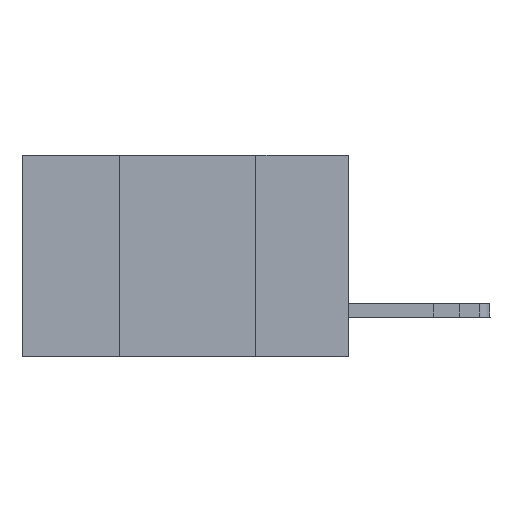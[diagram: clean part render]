
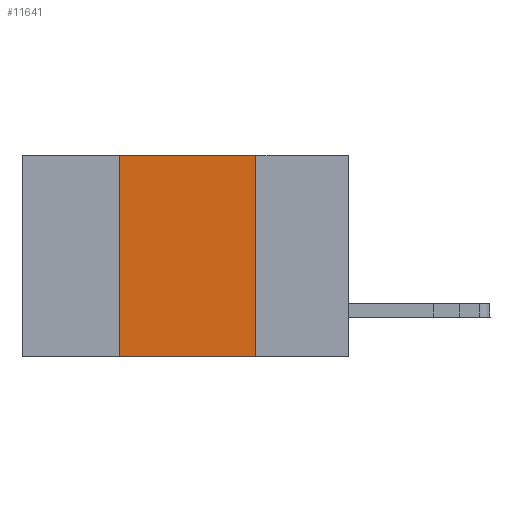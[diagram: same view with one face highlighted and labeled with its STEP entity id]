
A CAD part, left-side view. The second image highlights one B-rep face of the part: STEP entity #11641.
In plain terms, the highlighted planar face has unit normal (-1, 0, 0).
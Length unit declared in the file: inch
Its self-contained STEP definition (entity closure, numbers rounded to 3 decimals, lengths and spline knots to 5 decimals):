
#175 = ORIENTED_EDGE ( 'NONE', *, *, #22905, .F. ) ;
#768 = CARTESIAN_POINT ( 'NONE',  ( 0., 0.6, -0.37 ) ) ;
#1078 = VERTEX_POINT ( 'NONE', #2141 ) ;
#1504 = CARTESIAN_POINT ( 'NONE',  ( 0., 0.42, 0. ) ) ;
#1736 = ORIENTED_EDGE ( 'NONE', *, *, #4784, .T. ) ;
#2096 = PLANE ( 'NONE',  #23273 ) ;
#2141 = CARTESIAN_POINT ( 'NONE',  ( 0., 0.17, 0. ) ) ;
#2751 = VECTOR ( 'NONE', #10337, 39.37008 ) ;
#4326 = CARTESIAN_POINT ( 'NONE',  ( 0., 0.42, -0.37 ) ) ;
#4784 = EDGE_CURVE ( 'NONE', #15627, #7791, #23491, .T. ) ;
#4946 = EDGE_CURVE ( 'NONE', #1078, #7791, #5081, .T. ) ;
#5081 = LINE ( 'NONE', #23608, #14709 ) ;
#5235 = VECTOR ( 'NONE', #21622, 39.37008 ) ;
#6411 = ORIENTED_EDGE ( 'NONE', *, *, #6526, .F. ) ;
#6526 = EDGE_CURVE ( 'NONE', #13753, #1078, #7897, .T. ) ;
#7791 = VERTEX_POINT ( 'NONE', #24075 ) ;
#7897 = LINE ( 'NONE', #15511, #5235 ) ;
#8139 = CARTESIAN_POINT ( 'NONE',  ( 0., 0.6, 0. ) ) ;
#9649 = DIRECTION ( 'NONE',  ( 1., 0., 0. ) ) ;
#9808 = DIRECTION ( 'NONE',  ( 0., -1., 0. ) ) ;
#9970 = LINE ( 'NONE', #15951, #2751 ) ;
#10337 = DIRECTION ( 'NONE',  ( 0., 0., 1. ) ) ;
#11641 = ADVANCED_FACE ( 'NONE', ( #19132 ), #2096, .F. ) ;
#12657 = DIRECTION ( 'NONE',  ( 0., 0., -1. ) ) ;
#13753 = VERTEX_POINT ( 'NONE', #1504 ) ;
#14709 = VECTOR ( 'NONE', #12657, 39.37008 ) ;
#15511 = CARTESIAN_POINT ( 'NONE',  ( 0., 0.6, 0. ) ) ;
#15627 = VERTEX_POINT ( 'NONE', #4326 ) ;
#15951 = CARTESIAN_POINT ( 'NONE',  ( 0., 0.42, 0. ) ) ;
#16322 = VECTOR ( 'NONE', #9808, 39.37008 ) ;
#17953 = EDGE_LOOP ( 'NONE', ( #22990, #6411, #175, #1736 ) ) ;
#19132 = FACE_OUTER_BOUND ( 'NONE', #17953, .T. ) ;
#21360 = DIRECTION ( 'NONE',  ( 0., 0., -1. ) ) ;
#21622 = DIRECTION ( 'NONE',  ( 0., -1., 0. ) ) ;
#22905 = EDGE_CURVE ( 'NONE', #15627, #13753, #9970, .T. ) ;
#22990 = ORIENTED_EDGE ( 'NONE', *, *, #4946, .F. ) ;
#23273 = AXIS2_PLACEMENT_3D ( 'NONE', #8139, #9649, #21360 ) ;
#23491 = LINE ( 'NONE', #768, #16322 ) ;
#23608 = CARTESIAN_POINT ( 'NONE',  ( 0., 0.17, 0. ) ) ;
#24075 = CARTESIAN_POINT ( 'NONE',  ( 0., 0.17, -0.37 ) ) ;
